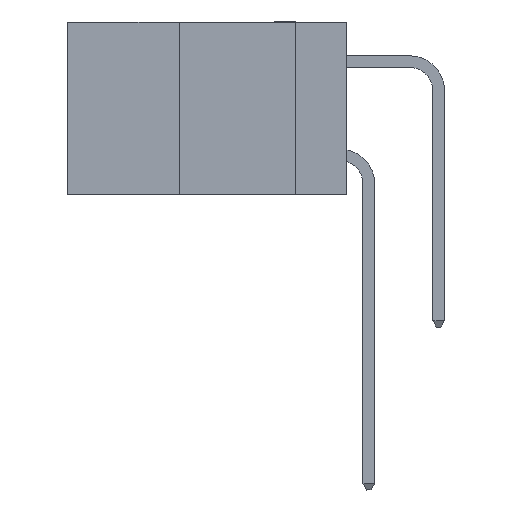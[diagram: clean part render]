
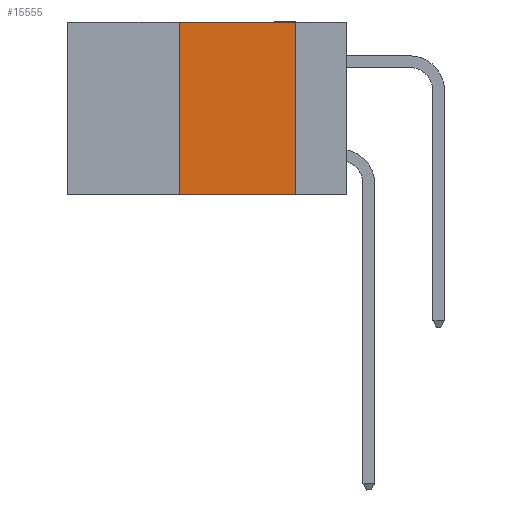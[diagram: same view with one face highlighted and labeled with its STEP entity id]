
A CAD part, left-side view. The second image highlights one B-rep face of the part: STEP entity #15555.
In plain terms, the highlighted planar face has unit normal (-1, 0, 0).
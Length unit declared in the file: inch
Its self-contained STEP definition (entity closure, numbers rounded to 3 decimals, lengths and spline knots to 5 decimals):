
#76 = EDGE_CURVE ( 'NONE', #779, #15819, #17534, .T. ) ;
#304 = VERTEX_POINT ( 'NONE', #12609 ) ;
#779 = VERTEX_POINT ( 'NONE', #12538 ) ;
#1063 = PLANE ( 'NONE',  #1139 ) ;
#1139 = AXIS2_PLACEMENT_3D ( 'NONE', #5893, #17984, #9050 ) ;
#1368 = CARTESIAN_POINT ( 'NONE',  ( 0., 0.11, 0. ) ) ;
#1495 = VECTOR ( 'NONE', #5033, 39.37008 ) ;
#2422 = LINE ( 'NONE', #1368, #14289 ) ;
#3925 = CARTESIAN_POINT ( 'NONE',  ( 0., 0.6, 0. ) ) ;
#5033 = DIRECTION ( 'NONE',  ( 0., 0., 1. ) ) ;
#5089 = CARTESIAN_POINT ( 'NONE',  ( 0., 0.36, 0. ) ) ;
#5737 = LINE ( 'NONE', #5089, #1495 ) ;
#5893 = CARTESIAN_POINT ( 'NONE',  ( 0., 0.6, 0. ) ) ;
#6000 = ORIENTED_EDGE ( 'NONE', *, *, #16020, .F. ) ;
#6751 = EDGE_CURVE ( 'NONE', #779, #17512, #5737, .T. ) ;
#8463 = ORIENTED_EDGE ( 'NONE', *, *, #15004, .F. ) ;
#9050 = DIRECTION ( 'NONE',  ( 0., 0., -1. ) ) ;
#10140 = ORIENTED_EDGE ( 'NONE', *, *, #76, .T. ) ;
#10415 = CARTESIAN_POINT ( 'NONE',  ( 0., 0.6, -0.37 ) ) ;
#10426 = CARTESIAN_POINT ( 'NONE',  ( 0., 0.36, 0. ) ) ;
#11675 = DIRECTION ( 'NONE',  ( 0., -1., 0. ) ) ;
#12538 = CARTESIAN_POINT ( 'NONE',  ( 0., 0.36, -0.37 ) ) ;
#12609 = CARTESIAN_POINT ( 'NONE',  ( 0., 0.11, 0. ) ) ;
#12661 = CARTESIAN_POINT ( 'NONE',  ( 0., 0.11, -0.37 ) ) ;
#13423 = VECTOR ( 'NONE', #17938, 39.37008 ) ;
#14239 = EDGE_LOOP ( 'NONE', ( #8463, #6000, #18051, #10140 ) ) ;
#14289 = VECTOR ( 'NONE', #16697, 39.37008 ) ;
#14469 = VECTOR ( 'NONE', #11675, 39.37008 ) ;
#14925 = LINE ( 'NONE', #3925, #14469 ) ;
#15004 = EDGE_CURVE ( 'NONE', #304, #15819, #2422, .T. ) ;
#15555 = ADVANCED_FACE ( 'NONE', ( #15854 ), #1063, .F. ) ;
#15819 = VERTEX_POINT ( 'NONE', #12661 ) ;
#15854 = FACE_OUTER_BOUND ( 'NONE', #14239, .T. ) ;
#16020 = EDGE_CURVE ( 'NONE', #17512, #304, #14925, .T. ) ;
#16697 = DIRECTION ( 'NONE',  ( 0., 0., -1. ) ) ;
#17512 = VERTEX_POINT ( 'NONE', #10426 ) ;
#17534 = LINE ( 'NONE', #10415, #13423 ) ;
#17938 = DIRECTION ( 'NONE',  ( 0., -1., 0. ) ) ;
#17984 = DIRECTION ( 'NONE',  ( 1., 0., 0. ) ) ;
#18051 = ORIENTED_EDGE ( 'NONE', *, *, #6751, .F. ) ;
